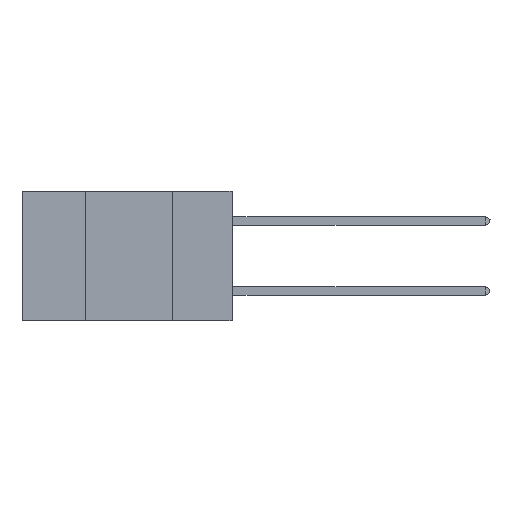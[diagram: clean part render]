
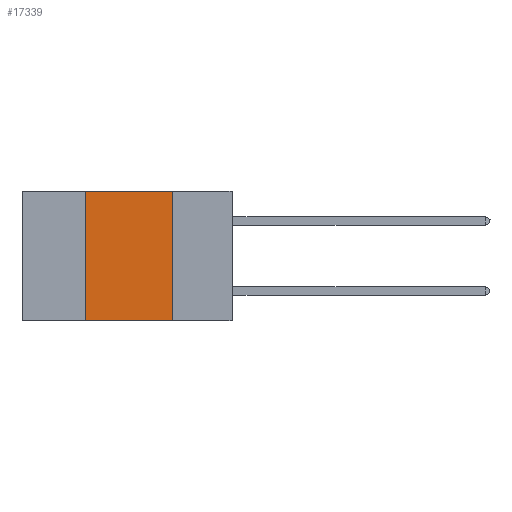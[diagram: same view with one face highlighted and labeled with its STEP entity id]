
A CAD part, left-side view. The second image highlights one B-rep face of the part: STEP entity #17339.
In plain terms, the highlighted planar face has unit normal (-1, 0, 0).
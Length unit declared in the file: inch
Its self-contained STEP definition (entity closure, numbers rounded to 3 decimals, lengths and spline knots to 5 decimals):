
#88 = DIRECTION ( 'NONE',  ( 1., 0., 0. ) ) ;
#1154 = EDGE_CURVE ( 'NONE', #18997, #4117, #10777, .T. ) ;
#1857 = PLANE ( 'NONE',  #18027 ) ;
#1983 = LINE ( 'NONE', #13844, #2528 ) ;
#2528 = VECTOR ( 'NONE', #19628, 39.37008 ) ;
#2682 = DIRECTION ( 'NONE',  ( 0., 0., 1. ) ) ;
#2862 = LINE ( 'NONE', #20147, #21749 ) ;
#3673 = EDGE_CURVE ( 'NONE', #18997, #17876, #1983, .T. ) ;
#3745 = VECTOR ( 'NONE', #2682, 39.37008 ) ;
#3978 = CARTESIAN_POINT ( 'NONE',  ( 0., 0.42, -0.37 ) ) ;
#4117 = VERTEX_POINT ( 'NONE', #17926 ) ;
#4985 = DIRECTION ( 'NONE',  ( 0., -1., 0. ) ) ;
#5478 = CARTESIAN_POINT ( 'NONE',  ( 0., 0.6, 0. ) ) ;
#6027 = DIRECTION ( 'NONE',  ( 0., 0., -1. ) ) ;
#6263 = ORIENTED_EDGE ( 'NONE', *, *, #3673, .T. ) ;
#6554 = CARTESIAN_POINT ( 'NONE',  ( 0., 0.17, 0. ) ) ;
#7864 = EDGE_CURVE ( 'NONE', #12032, #17876, #2862, .T. ) ;
#10584 = DIRECTION ( 'NONE',  ( 0., 0., -1. ) ) ;
#10635 = CARTESIAN_POINT ( 'NONE',  ( 0., 0.17, -0.37 ) ) ;
#10777 = LINE ( 'NONE', #18196, #3745 ) ;
#12032 = VERTEX_POINT ( 'NONE', #6554 ) ;
#12117 = ORIENTED_EDGE ( 'NONE', *, *, #1154, .F. ) ;
#13085 = ORIENTED_EDGE ( 'NONE', *, *, #16928, .F. ) ;
#13201 = VECTOR ( 'NONE', #4985, 39.37008 ) ;
#13402 = EDGE_LOOP ( 'NONE', ( #21182, #13085, #12117, #6263 ) ) ;
#13844 = CARTESIAN_POINT ( 'NONE',  ( 0., 0.6, -0.37 ) ) ;
#14936 = LINE ( 'NONE', #5478, #13201 ) ;
#16928 = EDGE_CURVE ( 'NONE', #4117, #12032, #14936, .T. ) ;
#17339 = ADVANCED_FACE ( 'NONE', ( #19133 ), #1857, .F. ) ;
#17876 = VERTEX_POINT ( 'NONE', #10635 ) ;
#17926 = CARTESIAN_POINT ( 'NONE',  ( 0., 0.42, 0. ) ) ;
#18027 = AXIS2_PLACEMENT_3D ( 'NONE', #21370, #88, #6027 ) ;
#18196 = CARTESIAN_POINT ( 'NONE',  ( 0., 0.42, 0. ) ) ;
#18997 = VERTEX_POINT ( 'NONE', #3978 ) ;
#19133 = FACE_OUTER_BOUND ( 'NONE', #13402, .T. ) ;
#19628 = DIRECTION ( 'NONE',  ( 0., -1., 0. ) ) ;
#20147 = CARTESIAN_POINT ( 'NONE',  ( 0., 0.17, 0. ) ) ;
#21182 = ORIENTED_EDGE ( 'NONE', *, *, #7864, .F. ) ;
#21370 = CARTESIAN_POINT ( 'NONE',  ( 0., 0.6, 0. ) ) ;
#21749 = VECTOR ( 'NONE', #10584, 39.37008 ) ;
